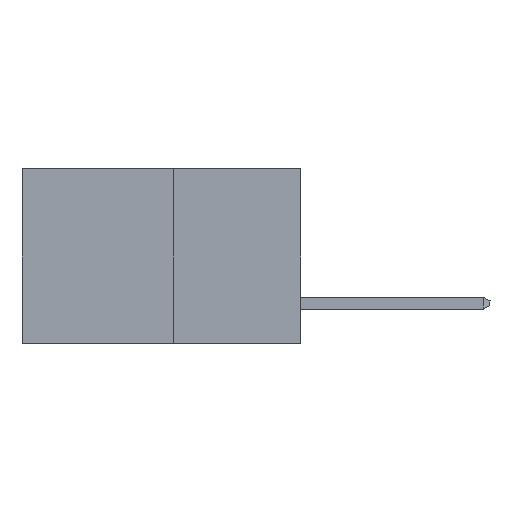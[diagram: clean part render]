
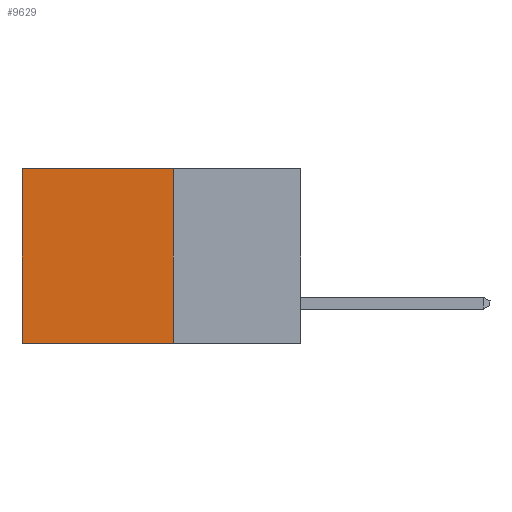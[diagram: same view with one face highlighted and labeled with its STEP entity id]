
A CAD part, left-side view. The second image highlights one B-rep face of the part: STEP entity #9629.
In plain terms, the highlighted planar face has unit normal (-1, 0, 0).
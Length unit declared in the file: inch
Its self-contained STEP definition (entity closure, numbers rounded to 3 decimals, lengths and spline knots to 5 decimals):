
#427 = VECTOR ( 'NONE', #4783, 39.37008 ) ;
#515 = EDGE_CURVE ( 'NONE', #8932, #2969, #796, .T. ) ;
#796 = LINE ( 'NONE', #3351, #5319 ) ;
#1311 = ORIENTED_EDGE ( 'NONE', *, *, #4078, .T. ) ;
#2228 = ORIENTED_EDGE ( 'NONE', *, *, #6714, .F. ) ;
#2937 = LINE ( 'NONE', #4649, #427 ) ;
#2969 = VERTEX_POINT ( 'NONE', #6218 ) ;
#3232 = DIRECTION ( 'NONE',  ( 1., 0., 0. ) ) ;
#3351 = CARTESIAN_POINT ( 'NONE',  ( 0.277, 0.27, 0. ) ) ;
#3459 = CARTESIAN_POINT ( 'NONE',  ( 0.277, 0.27, -0.37 ) ) ;
#3620 = CARTESIAN_POINT ( 'NONE',  ( 0.277, 0.59, -0.37 ) ) ;
#4078 = EDGE_CURVE ( 'NONE', #2969, #8529, #10353, .T. ) ;
#4649 = CARTESIAN_POINT ( 'NONE',  ( 0.277, 0.27, -0.37 ) ) ;
#4677 = CARTESIAN_POINT ( 'NONE',  ( 0.277, 0.27, -0.37 ) ) ;
#4783 = DIRECTION ( 'NONE',  ( 0., 1., 0. ) ) ;
#4855 = EDGE_CURVE ( 'NONE', #8932, #9090, #8128, .T. ) ;
#4935 = EDGE_LOOP ( 'NONE', ( #1311, #2228, #6860, #5828 ) ) ;
#4973 = AXIS2_PLACEMENT_3D ( 'NONE', #8186, #3232, #8974 ) ;
#5319 = VECTOR ( 'NONE', #7034, 39.37008 ) ;
#5484 = DIRECTION ( 'NONE',  ( 0., 0., -1. ) ) ;
#5828 = ORIENTED_EDGE ( 'NONE', *, *, #515, .T. ) ;
#6218 = CARTESIAN_POINT ( 'NONE',  ( 0.277, 0.59, 0. ) ) ;
#6714 = EDGE_CURVE ( 'NONE', #9090, #8529, #2937, .T. ) ;
#6860 = ORIENTED_EDGE ( 'NONE', *, *, #4855, .F. ) ;
#7034 = DIRECTION ( 'NONE',  ( 0., 1., 0. ) ) ;
#7411 = PLANE ( 'NONE',  #4973 ) ;
#7457 = DIRECTION ( 'NONE',  ( 0., 0., -1. ) ) ;
#8128 = LINE ( 'NONE', #4677, #9973 ) ;
#8186 = CARTESIAN_POINT ( 'NONE',  ( 0.277, 0.27, -0.37 ) ) ;
#8246 = VECTOR ( 'NONE', #5484, 39.37008 ) ;
#8529 = VERTEX_POINT ( 'NONE', #10934 ) ;
#8932 = VERTEX_POINT ( 'NONE', #8987 ) ;
#8974 = DIRECTION ( 'NONE',  ( 0., 0., -1. ) ) ;
#8987 = CARTESIAN_POINT ( 'NONE',  ( 0.277, 0.27, 0. ) ) ;
#9090 = VERTEX_POINT ( 'NONE', #3459 ) ;
#9629 = ADVANCED_FACE ( 'NONE', ( #10315 ), #7411, .F. ) ;
#9973 = VECTOR ( 'NONE', #7457, 39.37008 ) ;
#10315 = FACE_OUTER_BOUND ( 'NONE', #4935, .T. ) ;
#10353 = LINE ( 'NONE', #3620, #8246 ) ;
#10934 = CARTESIAN_POINT ( 'NONE',  ( 0.277, 0.59, -0.37 ) ) ;
